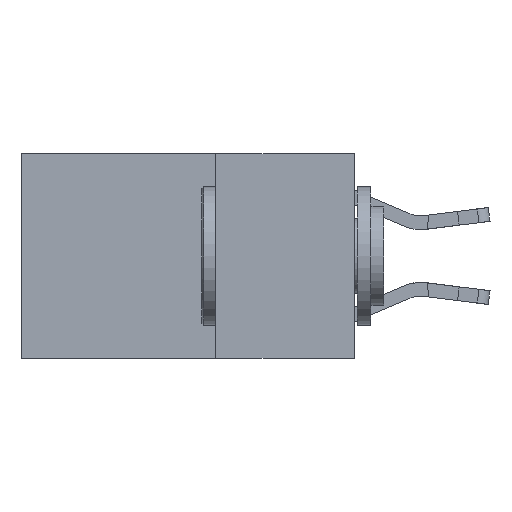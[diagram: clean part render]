
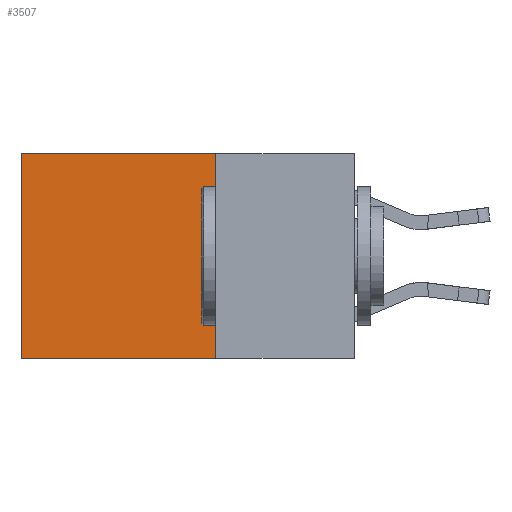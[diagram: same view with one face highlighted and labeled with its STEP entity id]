
A CAD part, left-side view. The second image highlights one B-rep face of the part: STEP entity #3507.
In plain terms, the highlighted planar face has unit normal (-1, 0, 0).
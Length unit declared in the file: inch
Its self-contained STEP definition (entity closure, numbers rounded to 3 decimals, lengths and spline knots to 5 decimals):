
#1035 = EDGE_CURVE ( 'NONE', #9542, #22734, #2719, .T. ) ;
#1870 = VECTOR ( 'NONE', #13853, 39.37008 ) ;
#2016 = CARTESIAN_POINT ( 'NONE',  ( 0.2625, 0.25, -0.37 ) ) ;
#2719 = LINE ( 'NONE', #10368, #23407 ) ;
#3233 = ORIENTED_EDGE ( 'NONE', *, *, #4578, .T. ) ;
#3373 = CARTESIAN_POINT ( 'NONE',  ( 0.2625, 0.6, 0. ) ) ;
#3507 = ADVANCED_FACE ( 'NONE', ( #16448 ), #5079, .F. ) ;
#4578 = EDGE_CURVE ( 'NONE', #9542, #11163, #8120, .T. ) ;
#4822 = DIRECTION ( 'NONE',  ( 0., 0., -1. ) ) ;
#5079 = PLANE ( 'NONE',  #8554 ) ;
#6472 = VECTOR ( 'NONE', #14906, 39.37008 ) ;
#6721 = DIRECTION ( 'NONE',  ( 1., 0., 0. ) ) ;
#7716 = ORIENTED_EDGE ( 'NONE', *, *, #18027, .F. ) ;
#8120 = LINE ( 'NONE', #23343, #1870 ) ;
#8138 = DIRECTION ( 'NONE',  ( 0., 0., -1. ) ) ;
#8554 = AXIS2_PLACEMENT_3D ( 'NONE', #10944, #6721, #4822 ) ;
#9542 = VERTEX_POINT ( 'NONE', #23434 ) ;
#10181 = CARTESIAN_POINT ( 'NONE',  ( 0.2625, 0.25, -0.37 ) ) ;
#10368 = CARTESIAN_POINT ( 'NONE',  ( 0.2625, 0.25, 0. ) ) ;
#10944 = CARTESIAN_POINT ( 'NONE',  ( 0.2625, 0.25, 0. ) ) ;
#11163 = VERTEX_POINT ( 'NONE', #23728 ) ;
#12189 = EDGE_CURVE ( 'NONE', #11163, #18886, #20517, .T. ) ;
#13853 = DIRECTION ( 'NONE',  ( 0., 1., 0. ) ) ;
#14906 = DIRECTION ( 'NONE',  ( 0., 0., -1. ) ) ;
#15199 = LINE ( 'NONE', #2016, #17533 ) ;
#16448 = FACE_OUTER_BOUND ( 'NONE', #22281, .T. ) ;
#17533 = VECTOR ( 'NONE', #20692, 39.37008 ) ;
#18027 = EDGE_CURVE ( 'NONE', #22734, #18886, #15199, .T. ) ;
#18886 = VERTEX_POINT ( 'NONE', #23070 ) ;
#20061 = ORIENTED_EDGE ( 'NONE', *, *, #1035, .F. ) ;
#20517 = LINE ( 'NONE', #3373, #6472 ) ;
#20692 = DIRECTION ( 'NONE',  ( 0., 1., 0. ) ) ;
#22281 = EDGE_LOOP ( 'NONE', ( #23485, #7716, #20061, #3233 ) ) ;
#22734 = VERTEX_POINT ( 'NONE', #10181 ) ;
#23070 = CARTESIAN_POINT ( 'NONE',  ( 0.2625, 0.6, -0.37 ) ) ;
#23343 = CARTESIAN_POINT ( 'NONE',  ( 0.2625, 0.25, 0. ) ) ;
#23407 = VECTOR ( 'NONE', #8138, 39.37008 ) ;
#23434 = CARTESIAN_POINT ( 'NONE',  ( 0.2625, 0.25, 0. ) ) ;
#23485 = ORIENTED_EDGE ( 'NONE', *, *, #12189, .T. ) ;
#23728 = CARTESIAN_POINT ( 'NONE',  ( 0.2625, 0.6, 0. ) ) ;
